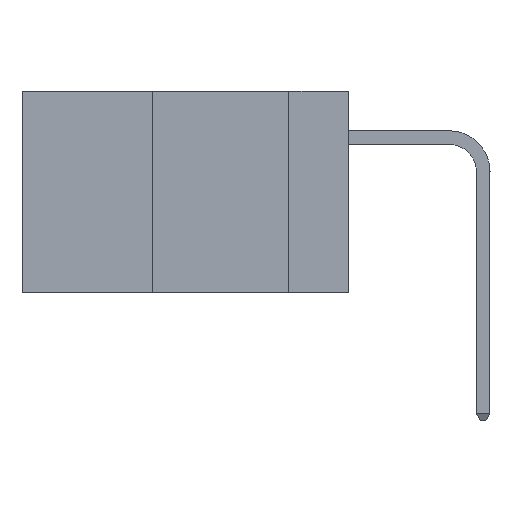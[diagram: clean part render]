
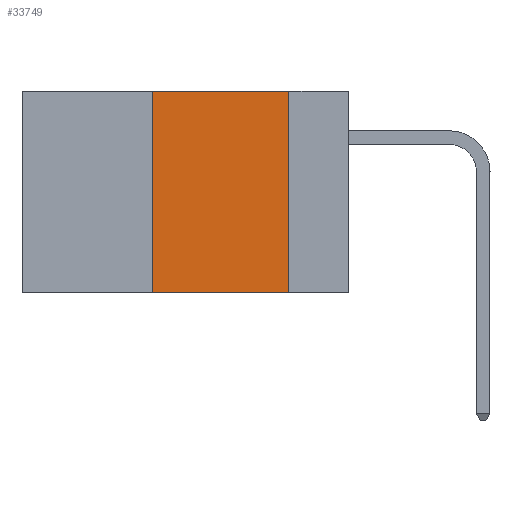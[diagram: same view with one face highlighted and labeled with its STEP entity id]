
A CAD part, left-side view. The second image highlights one B-rep face of the part: STEP entity #33749.
In plain terms, the highlighted planar face has unit normal (-1, 0, 0).
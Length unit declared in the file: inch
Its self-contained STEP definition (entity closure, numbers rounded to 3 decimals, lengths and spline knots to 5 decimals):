
#63 = CARTESIAN_POINT ( 'NONE',  ( 0., 0.11, 0. ) ) ;
#3962 = LINE ( 'NONE', #63, #10611 ) ;
#5830 = DIRECTION ( 'NONE',  ( 0., 0., 1. ) ) ;
#5903 = CARTESIAN_POINT ( 'NONE',  ( 0., 0.6, -0.37 ) ) ;
#6102 = CARTESIAN_POINT ( 'NONE',  ( 0., 0.6, 0. ) ) ;
#6150 = ORIENTED_EDGE ( 'NONE', *, *, #30751, .F. ) ;
#8021 = DIRECTION ( 'NONE',  ( 0., -1., 0. ) ) ;
#8951 = DIRECTION ( 'NONE',  ( 1., 0., 0. ) ) ;
#10527 = AXIS2_PLACEMENT_3D ( 'NONE', #6102, #8951, #28796 ) ;
#10611 = VECTOR ( 'NONE', #31201, 39.37008 ) ;
#11760 = EDGE_LOOP ( 'NONE', ( #31855, #26520, #6150, #22577 ) ) ;
#11865 = VERTEX_POINT ( 'NONE', #30178 ) ;
#13160 = VERTEX_POINT ( 'NONE', #33078 ) ;
#13953 = VERTEX_POINT ( 'NONE', #16380 ) ;
#15063 = EDGE_CURVE ( 'NONE', #11865, #13953, #24487, .T. ) ;
#16064 = VECTOR ( 'NONE', #31474, 39.37008 ) ;
#16380 = CARTESIAN_POINT ( 'NONE',  ( 0., 0.11, -0.37 ) ) ;
#19842 = LINE ( 'NONE', #19971, #27394 ) ;
#19971 = CARTESIAN_POINT ( 'NONE',  ( 0., 0.36, 0. ) ) ;
#22577 = ORIENTED_EDGE ( 'NONE', *, *, #15063, .T. ) ;
#24487 = LINE ( 'NONE', #5903, #16064 ) ;
#25240 = CARTESIAN_POINT ( 'NONE',  ( 0., 0.11, 0. ) ) ;
#25675 = EDGE_CURVE ( 'NONE', #13160, #26273, #29141, .T. ) ;
#25936 = PLANE ( 'NONE',  #10527 ) ;
#26273 = VERTEX_POINT ( 'NONE', #25240 ) ;
#26520 = ORIENTED_EDGE ( 'NONE', *, *, #25675, .F. ) ;
#26895 = FACE_OUTER_BOUND ( 'NONE', #11760, .T. ) ;
#27359 = VECTOR ( 'NONE', #8021, 39.37008 ) ;
#27394 = VECTOR ( 'NONE', #5830, 39.37008 ) ;
#27894 = CARTESIAN_POINT ( 'NONE',  ( 0., 0.6, 0. ) ) ;
#28796 = DIRECTION ( 'NONE',  ( 0., 0., -1. ) ) ;
#29141 = LINE ( 'NONE', #27894, #27359 ) ;
#30025 = EDGE_CURVE ( 'NONE', #26273, #13953, #3962, .T. ) ;
#30178 = CARTESIAN_POINT ( 'NONE',  ( 0., 0.36, -0.37 ) ) ;
#30751 = EDGE_CURVE ( 'NONE', #11865, #13160, #19842, .T. ) ;
#31201 = DIRECTION ( 'NONE',  ( 0., 0., -1. ) ) ;
#31474 = DIRECTION ( 'NONE',  ( 0., -1., 0. ) ) ;
#31855 = ORIENTED_EDGE ( 'NONE', *, *, #30025, .F. ) ;
#33078 = CARTESIAN_POINT ( 'NONE',  ( 0., 0.36, 0. ) ) ;
#33749 = ADVANCED_FACE ( 'NONE', ( #26895 ), #25936, .F. ) ;
